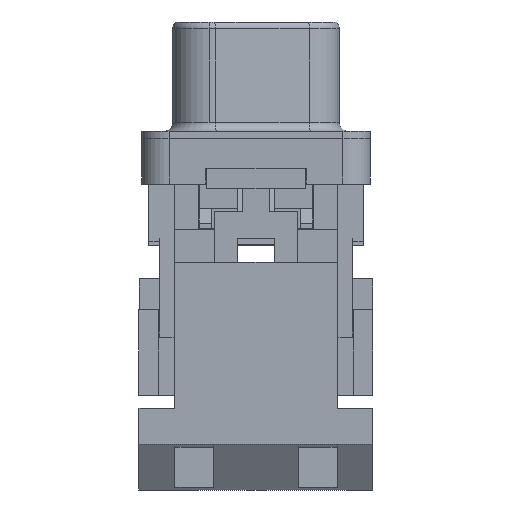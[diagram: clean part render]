
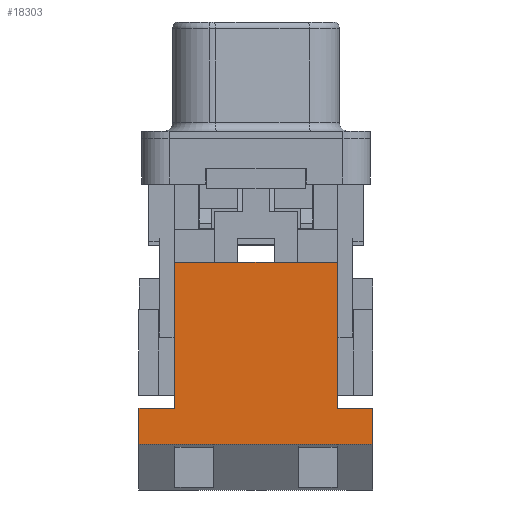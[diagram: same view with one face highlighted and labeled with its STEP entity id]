
A CAD part, left-side view. The second image highlights one B-rep face of the part: STEP entity #18303.
In plain terms, the highlighted planar face has unit normal (-1, 0, 0).
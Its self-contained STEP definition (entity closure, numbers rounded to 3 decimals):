
#27 = CARTESIAN_POINT ( 'NONE',  ( 3.245, -6.425, -14.8 ) ) ;
#250 = VERTEX_POINT ( 'NONE', #12936 ) ;
#1092 = DIRECTION ( 'NONE',  ( 0., 0., -1. ) ) ;
#1568 = VECTOR ( 'NONE', #9031, 1000. ) ;
#2094 = VECTOR ( 'NONE', #25880, 1000. ) ;
#2889 = VECTOR ( 'NONE', #22241, 1000. ) ;
#3176 = VERTEX_POINT ( 'NONE', #16156 ) ;
#3542 = ORIENTED_EDGE ( 'NONE', *, *, #25124, .F. ) ;
#4052 = DIRECTION ( 'NONE',  ( 0., -1., 0. ) ) ;
#4616 = CARTESIAN_POINT ( 'NONE',  ( 3.245, 4.45, -6.8 ) ) ;
#5289 = LINE ( 'NONE', #22602, #2094 ) ;
#5439 = CARTESIAN_POINT ( 'NONE',  ( 3.245, -6.425, -15.3 ) ) ;
#5645 = EDGE_CURVE ( 'NONE', #250, #16684, #24639, .T. ) ;
#8317 = EDGE_CURVE ( 'NONE', #3176, #12963, #35262, .T. ) ;
#9031 = DIRECTION ( 'NONE',  ( 0., 0., -1. ) ) ;
#10697 = CARTESIAN_POINT ( 'NONE',  ( 3.245, 6.425, -14.8 ) ) ;
#11015 = DIRECTION ( 'NONE',  ( 0., 0., -1. ) ) ;
#11861 = AXIS2_PLACEMENT_3D ( 'NONE', #5439, #26009, #11015 ) ;
#11927 = LINE ( 'NONE', #15701, #1568 ) ;
#12628 = LINE ( 'NONE', #24358, #21996 ) ;
#12936 = CARTESIAN_POINT ( 'NONE',  ( 3.245, 6.425, -14.8 ) ) ;
#12963 = VERTEX_POINT ( 'NONE', #19765 ) ;
#13775 = DIRECTION ( 'NONE',  ( 0., 0., -1. ) ) ;
#13821 = VERTEX_POINT ( 'NONE', #31979 ) ;
#13958 = LINE ( 'NONE', #37221, #36190 ) ;
#15558 = ORIENTED_EDGE ( 'NONE', *, *, #5645, .F. ) ;
#15701 = CARTESIAN_POINT ( 'NONE',  ( 3.245, 4.45, -6.8 ) ) ;
#16156 = CARTESIAN_POINT ( 'NONE',  ( 3.245, -6.425, -16.8 ) ) ;
#16256 = VERTEX_POINT ( 'NONE', #28208 ) ;
#16335 = LINE ( 'NONE', #4616, #32495 ) ;
#16684 = VERTEX_POINT ( 'NONE', #25079 ) ;
#17676 = VECTOR ( 'NONE', #34687, 1000. ) ;
#17996 = EDGE_CURVE ( 'NONE', #24543, #16256, #5289, .T. ) ;
#18303 = ADVANCED_FACE ( 'NONE', ( #22746 ), #19855, .F. ) ;
#18656 = DIRECTION ( 'NONE',  ( 0., -1., 0. ) ) ;
#19061 = CARTESIAN_POINT ( 'NONE',  ( 3.245, 6.425, -14.8 ) ) ;
#19765 = CARTESIAN_POINT ( 'NONE',  ( 3.245, 6.425, -16.8 ) ) ;
#19855 = PLANE ( 'NONE',  #11861 ) ;
#20020 = ORIENTED_EDGE ( 'NONE', *, *, #29962, .T. ) ;
#21495 = EDGE_CURVE ( 'NONE', #13821, #24543, #16335, .T. ) ;
#21747 = CARTESIAN_POINT ( 'NONE',  ( 3.245, -4.45, -6.8 ) ) ;
#21996 = VECTOR ( 'NONE', #1092, 1000. ) ;
#22241 = DIRECTION ( 'NONE',  ( 0., -1., 0. ) ) ;
#22602 = CARTESIAN_POINT ( 'NONE',  ( 3.245, -4.45, -6.8 ) ) ;
#22746 = FACE_OUTER_BOUND ( 'NONE', #27604, .T. ) ;
#24176 = ORIENTED_EDGE ( 'NONE', *, *, #21495, .F. ) ;
#24358 = CARTESIAN_POINT ( 'NONE',  ( 3.245, 6.425, -15.3 ) ) ;
#24543 = VERTEX_POINT ( 'NONE', #21747 ) ;
#24639 = LINE ( 'NONE', #19061, #37722 ) ;
#25079 = CARTESIAN_POINT ( 'NONE',  ( 3.245, 4.45, -14.8 ) ) ;
#25124 = EDGE_CURVE ( 'NONE', #31024, #3176, #13958, .T. ) ;
#25327 = LINE ( 'NONE', #10697, #2889 ) ;
#25880 = DIRECTION ( 'NONE',  ( 0., 0., -1. ) ) ;
#26009 = DIRECTION ( 'NONE',  ( 1., 0., 0. ) ) ;
#27604 = EDGE_LOOP ( 'NONE', ( #37816, #29219, #3542, #29373, #29187, #24176, #20020, #15558 ) ) ;
#28208 = CARTESIAN_POINT ( 'NONE',  ( 3.245, -4.45, -14.8 ) ) ;
#29187 = ORIENTED_EDGE ( 'NONE', *, *, #17996, .F. ) ;
#29219 = ORIENTED_EDGE ( 'NONE', *, *, #8317, .F. ) ;
#29373 = ORIENTED_EDGE ( 'NONE', *, *, #31644, .F. ) ;
#29962 = EDGE_CURVE ( 'NONE', #13821, #16684, #11927, .T. ) ;
#31024 = VERTEX_POINT ( 'NONE', #27 ) ;
#31644 = EDGE_CURVE ( 'NONE', #16256, #31024, #25327, .T. ) ;
#31817 = CARTESIAN_POINT ( 'NONE',  ( 3.245, -6.425, -16.8 ) ) ;
#31979 = CARTESIAN_POINT ( 'NONE',  ( 3.245, 4.45, -6.8 ) ) ;
#32495 = VECTOR ( 'NONE', #18656, 1000. ) ;
#34418 = EDGE_CURVE ( 'NONE', #250, #12963, #12628, .T. ) ;
#34687 = DIRECTION ( 'NONE',  ( 0., 1., 0. ) ) ;
#35262 = LINE ( 'NONE', #31817, #17676 ) ;
#36190 = VECTOR ( 'NONE', #13775, 1000. ) ;
#37221 = CARTESIAN_POINT ( 'NONE',  ( 3.245, -6.425, -15.3 ) ) ;
#37722 = VECTOR ( 'NONE', #4052, 1000. ) ;
#37816 = ORIENTED_EDGE ( 'NONE', *, *, #34418, .T. ) ;
